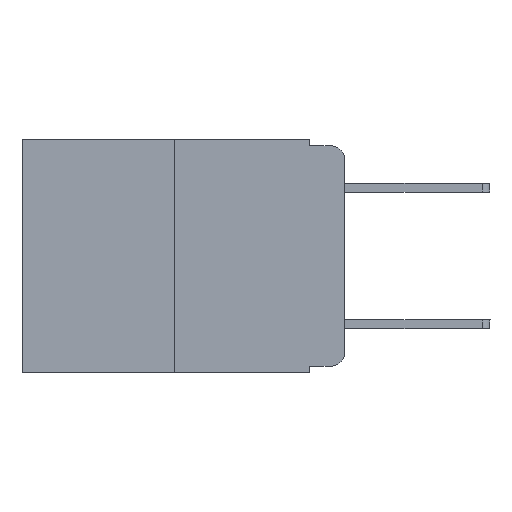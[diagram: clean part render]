
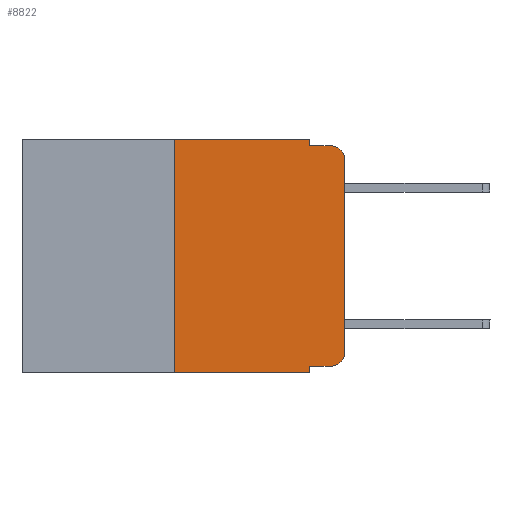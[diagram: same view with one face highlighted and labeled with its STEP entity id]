
A CAD part, left-side view. The second image highlights one B-rep face of the part: STEP entity #8822.
In plain terms, the highlighted planar face has unit normal (-1, 0, 0).
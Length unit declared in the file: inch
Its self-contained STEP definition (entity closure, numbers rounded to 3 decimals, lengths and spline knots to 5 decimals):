
#20 = CARTESIAN_POINT ( 'NONE',  ( 0., 0.25, 0. ) ) ;
#230 = VECTOR ( 'NONE', #19090, 39.37008 ) ;
#374 = DIRECTION ( 'NONE',  ( 0., -1., 0. ) ) ;
#716 = CIRCLE ( 'NONE', #10467, 0.02 ) ;
#809 = DIRECTION ( 'NONE',  ( -1., 0., 0. ) ) ;
#1177 = CARTESIAN_POINT ( 'NONE',  ( 0., 0.051, -0.343 ) ) ;
#2007 = DIRECTION ( 'NONE',  ( 0., -1., 0. ) ) ;
#2241 = LINE ( 'NONE', #14576, #6454 ) ;
#2823 = VERTEX_POINT ( 'NONE', #1177 ) ;
#2981 = DIRECTION ( 'NONE',  ( 0., 0., -1. ) ) ;
#3208 = VERTEX_POINT ( 'NONE', #13344 ) ;
#3420 = EDGE_CURVE ( 'NONE', #3208, #20200, #14461, .T. ) ;
#3810 = CARTESIAN_POINT ( 'NONE',  ( 0., 0.051, -0.333 ) ) ;
#3940 = AXIS2_PLACEMENT_3D ( 'NONE', #5846, #9492, #21729 ) ;
#3949 = VERTEX_POINT ( 'NONE', #14542 ) ;
#4527 = VECTOR ( 'NONE', #9292, 39.37008 ) ;
#4649 = VECTOR ( 'NONE', #2007, 39.37008 ) ;
#4697 = EDGE_CURVE ( 'NONE', #16609, #20200, #716, .T. ) ;
#4792 = LINE ( 'NONE', #7722, #18830 ) ;
#5461 = AXIS2_PLACEMENT_3D ( 'NONE', #14966, #809, #11401 ) ;
#5846 = CARTESIAN_POINT ( 'NONE',  ( 0., 0.473, 0. ) ) ;
#6003 = ORIENTED_EDGE ( 'NONE', *, *, #16509, .T. ) ;
#6454 = VECTOR ( 'NONE', #374, 39.37008 ) ;
#6555 = CARTESIAN_POINT ( 'NONE',  ( 0., 0., 0. ) ) ;
#6794 = EDGE_LOOP ( 'NONE', ( #6003, #10322, #19365, #15552, #21613, #11631, #16526, #19099, #22420, #19116 ) ) ;
#6850 = VERTEX_POINT ( 'NONE', #9998 ) ;
#6883 = LINE ( 'NONE', #9115, #4649 ) ;
#7421 = CIRCLE ( 'NONE', #5461, 0.02 ) ;
#7482 = CARTESIAN_POINT ( 'NONE',  ( 0., 0.02, -0.333 ) ) ;
#7618 = CARTESIAN_POINT ( 'NONE',  ( 0., 0.02, -0.01 ) ) ;
#7722 = CARTESIAN_POINT ( 'NONE',  ( 0., 0.473, 0. ) ) ;
#8471 = VECTOR ( 'NONE', #2981, 39.37008 ) ;
#8475 = EDGE_CURVE ( 'NONE', #3949, #3208, #18004, .T. ) ;
#8639 = DIRECTION ( 'NONE',  ( 0., -1., 0. ) ) ;
#8657 = VERTEX_POINT ( 'NONE', #3810 ) ;
#8822 = ADVANCED_FACE ( 'NONE', ( #11541 ), #20234, .F. ) ;
#9115 = CARTESIAN_POINT ( 'NONE',  ( 0., 0.473, -0.343 ) ) ;
#9292 = DIRECTION ( 'NONE',  ( 0., 0., 1. ) ) ;
#9492 = DIRECTION ( 'NONE',  ( 1., 0., 0. ) ) ;
#9504 = DIRECTION ( 'NONE',  ( 0., -1., 0. ) ) ;
#9705 = EDGE_CURVE ( 'NONE', #14041, #21356, #18558, .T. ) ;
#9998 = CARTESIAN_POINT ( 'NONE',  ( 0., 0., -0.313 ) ) ;
#10078 = CARTESIAN_POINT ( 'NONE',  ( 0., 0.051, 0. ) ) ;
#10322 = ORIENTED_EDGE ( 'NONE', *, *, #4697, .T. ) ;
#10467 = AXIS2_PLACEMENT_3D ( 'NONE', #15595, #22808, #12040 ) ;
#11401 = DIRECTION ( 'NONE',  ( 0., 0., -1. ) ) ;
#11541 = FACE_OUTER_BOUND ( 'NONE', #6794, .T. ) ;
#11631 = ORIENTED_EDGE ( 'NONE', *, *, #9705, .F. ) ;
#11822 = VECTOR ( 'NONE', #20764, 39.37008 ) ;
#12040 = DIRECTION ( 'NONE',  ( 0., 0., -1. ) ) ;
#12077 = CARTESIAN_POINT ( 'NONE',  ( 0., 0.051, -0.01 ) ) ;
#12290 = EDGE_CURVE ( 'NONE', #14041, #2823, #6883, .T. ) ;
#13344 = CARTESIAN_POINT ( 'NONE',  ( 0., 0.051, -0.01 ) ) ;
#13882 = CARTESIAN_POINT ( 'NONE',  ( 0., 0., -0.03 ) ) ;
#14041 = VERTEX_POINT ( 'NONE', #14705 ) ;
#14075 = EDGE_CURVE ( 'NONE', #21356, #3949, #4792, .T. ) ;
#14461 = LINE ( 'NONE', #12077, #20626 ) ;
#14542 = CARTESIAN_POINT ( 'NONE',  ( 0., 0.051, 0. ) ) ;
#14576 = CARTESIAN_POINT ( 'NONE',  ( 0., 0.051, -0.333 ) ) ;
#14705 = CARTESIAN_POINT ( 'NONE',  ( 0., 0.25, -0.343 ) ) ;
#14966 = CARTESIAN_POINT ( 'NONE',  ( 0., 0.02, -0.313 ) ) ;
#15391 = CARTESIAN_POINT ( 'NONE',  ( 0., 0.051, 0. ) ) ;
#15552 = ORIENTED_EDGE ( 'NONE', *, *, #8475, .F. ) ;
#15595 = CARTESIAN_POINT ( 'NONE',  ( 0., 0.02, -0.03 ) ) ;
#16509 = EDGE_CURVE ( 'NONE', #6850, #16609, #20074, .T. ) ;
#16526 = ORIENTED_EDGE ( 'NONE', *, *, #12290, .T. ) ;
#16609 = VERTEX_POINT ( 'NONE', #13882 ) ;
#17190 = LINE ( 'NONE', #15391, #11822 ) ;
#18004 = LINE ( 'NONE', #10078, #8471 ) ;
#18275 = VERTEX_POINT ( 'NONE', #7482 ) ;
#18558 = LINE ( 'NONE', #20021, #4527 ) ;
#18830 = VECTOR ( 'NONE', #9504, 39.37008 ) ;
#19090 = DIRECTION ( 'NONE',  ( 0., 0., 1. ) ) ;
#19099 = ORIENTED_EDGE ( 'NONE', *, *, #20578, .F. ) ;
#19116 = ORIENTED_EDGE ( 'NONE', *, *, #19179, .T. ) ;
#19179 = EDGE_CURVE ( 'NONE', #18275, #6850, #7421, .T. ) ;
#19365 = ORIENTED_EDGE ( 'NONE', *, *, #3420, .F. ) ;
#20021 = CARTESIAN_POINT ( 'NONE',  ( 0., 0.25, 0. ) ) ;
#20074 = LINE ( 'NONE', #6555, #230 ) ;
#20200 = VERTEX_POINT ( 'NONE', #7618 ) ;
#20234 = PLANE ( 'NONE',  #3940 ) ;
#20578 = EDGE_CURVE ( 'NONE', #8657, #2823, #17190, .T. ) ;
#20626 = VECTOR ( 'NONE', #8639, 39.37008 ) ;
#20764 = DIRECTION ( 'NONE',  ( 0., 0., -1. ) ) ;
#21356 = VERTEX_POINT ( 'NONE', #20 ) ;
#21613 = ORIENTED_EDGE ( 'NONE', *, *, #14075, .F. ) ;
#21729 = DIRECTION ( 'NONE',  ( 0., 0., -1. ) ) ;
#22417 = EDGE_CURVE ( 'NONE', #8657, #18275, #2241, .T. ) ;
#22420 = ORIENTED_EDGE ( 'NONE', *, *, #22417, .T. ) ;
#22808 = DIRECTION ( 'NONE',  ( -1., 0., 0. ) ) ;
